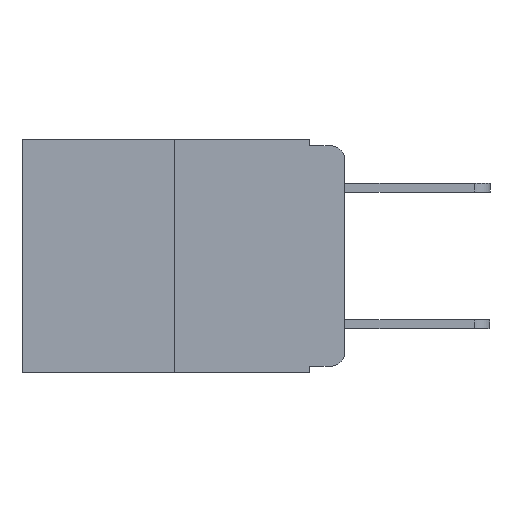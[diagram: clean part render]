
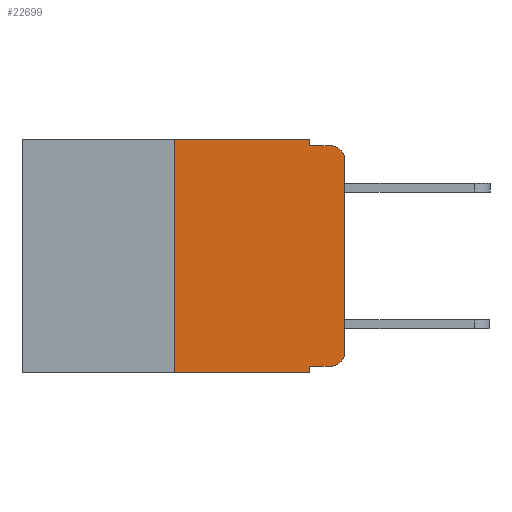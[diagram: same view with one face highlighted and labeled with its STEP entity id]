
A CAD part, left-side view. The second image highlights one B-rep face of the part: STEP entity #22699.
In plain terms, the highlighted planar face has unit normal (-1, 0, 0).
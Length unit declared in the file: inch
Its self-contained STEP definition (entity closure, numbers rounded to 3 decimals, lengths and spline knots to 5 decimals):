
#502 = DIRECTION ( 'NONE',  ( 0., -1., 0. ) ) ;
#968 = LINE ( 'NONE', #11239, #16253 ) ;
#1039 = CARTESIAN_POINT ( 'NONE',  ( 0., 0., -0.313 ) ) ;
#1352 = LINE ( 'NONE', #9816, #16007 ) ;
#1922 = LINE ( 'NONE', #12638, #11921 ) ;
#2007 = AXIS2_PLACEMENT_3D ( 'NONE', #10311, #23883, #12305 ) ;
#2706 = VECTOR ( 'NONE', #15380, 39.37008 ) ;
#2947 = ORIENTED_EDGE ( 'NONE', *, *, #20778, .T. ) ;
#3689 = VERTEX_POINT ( 'NONE', #8313 ) ;
#4048 = AXIS2_PLACEMENT_3D ( 'NONE', #19145, #7368, #21078 ) ;
#4637 = CARTESIAN_POINT ( 'NONE',  ( 0., 0.25, 0. ) ) ;
#5293 = LINE ( 'NONE', #9730, #15257 ) ;
#5774 = DIRECTION ( 'NONE',  ( 0., 0., -1. ) ) ;
#6338 = VERTEX_POINT ( 'NONE', #1039 ) ;
#7019 = ORIENTED_EDGE ( 'NONE', *, *, #24613, .T. ) ;
#7368 = DIRECTION ( 'NONE',  ( -1., 0., 0. ) ) ;
#7663 = EDGE_CURVE ( 'NONE', #12164, #6338, #9900, .T. ) ;
#8277 = EDGE_LOOP ( 'NONE', ( #7019, #2947, #14176, #24402, #10771, #17253, #13262, #8596, #19635, #24722 ) ) ;
#8313 = CARTESIAN_POINT ( 'NONE',  ( 0., 0.25, -0.343 ) ) ;
#8409 = VECTOR ( 'NONE', #10674, 39.37008 ) ;
#8506 = VERTEX_POINT ( 'NONE', #14765 ) ;
#8596 = ORIENTED_EDGE ( 'NONE', *, *, #14300, .F. ) ;
#8674 = VERTEX_POINT ( 'NONE', #11205 ) ;
#9271 = VECTOR ( 'NONE', #502, 39.37008 ) ;
#9400 = CARTESIAN_POINT ( 'NONE',  ( 0., 0., 0. ) ) ;
#9730 = CARTESIAN_POINT ( 'NONE',  ( 0., 0.473, 0. ) ) ;
#9816 = CARTESIAN_POINT ( 'NONE',  ( 0., 0.051, -0.333 ) ) ;
#9887 = LINE ( 'NONE', #12504, #9271 ) ;
#9900 = CIRCLE ( 'NONE', #2007, 0.02 ) ;
#10311 = CARTESIAN_POINT ( 'NONE',  ( 0., 0.02, -0.313 ) ) ;
#10498 = LINE ( 'NONE', #20859, #20245 ) ;
#10674 = DIRECTION ( 'NONE',  ( 0., 0., 1. ) ) ;
#10771 = ORIENTED_EDGE ( 'NONE', *, *, #15335, .F. ) ;
#11205 = CARTESIAN_POINT ( 'NONE',  ( 0., 0.051, -0.333 ) ) ;
#11239 = CARTESIAN_POINT ( 'NONE',  ( 0., 0.051, -0.01 ) ) ;
#11692 = CARTESIAN_POINT ( 'NONE',  ( 0., 0.473, 0. ) ) ;
#11721 = DIRECTION ( 'NONE',  ( 0., -1., 0. ) ) ;
#11921 = VECTOR ( 'NONE', #22449, 39.37008 ) ;
#12164 = VERTEX_POINT ( 'NONE', #17006 ) ;
#12305 = DIRECTION ( 'NONE',  ( 0., 0., -1. ) ) ;
#12504 = CARTESIAN_POINT ( 'NONE',  ( 0., 0.473, -0.343 ) ) ;
#12511 = CARTESIAN_POINT ( 'NONE',  ( 0., 0., -0.03 ) ) ;
#12638 = CARTESIAN_POINT ( 'NONE',  ( 0., 0.051, 0. ) ) ;
#12680 = VERTEX_POINT ( 'NONE', #12511 ) ;
#12684 = LINE ( 'NONE', #9400, #2706 ) ;
#12969 = EDGE_CURVE ( 'NONE', #8674, #12164, #1352, .T. ) ;
#13262 = ORIENTED_EDGE ( 'NONE', *, *, #24957, .T. ) ;
#13897 = VERTEX_POINT ( 'NONE', #17391 ) ;
#14028 = VERTEX_POINT ( 'NONE', #15843 ) ;
#14176 = ORIENTED_EDGE ( 'NONE', *, *, #19496, .F. ) ;
#14300 = EDGE_CURVE ( 'NONE', #8674, #8506, #1922, .T. ) ;
#14406 = VERTEX_POINT ( 'NONE', #22615 ) ;
#14765 = CARTESIAN_POINT ( 'NONE',  ( 0., 0.051, -0.343 ) ) ;
#15257 = VECTOR ( 'NONE', #11721, 39.37008 ) ;
#15335 = EDGE_CURVE ( 'NONE', #13897, #14406, #5293, .T. ) ;
#15380 = DIRECTION ( 'NONE',  ( 0., 0., 1. ) ) ;
#15629 = EDGE_CURVE ( 'NONE', #3689, #13897, #23933, .T. ) ;
#15679 = PLANE ( 'NONE',  #19598 ) ;
#15843 = CARTESIAN_POINT ( 'NONE',  ( 0., 0.051, -0.01 ) ) ;
#16007 = VECTOR ( 'NONE', #17735, 39.37008 ) ;
#16253 = VECTOR ( 'NONE', #22876, 39.37008 ) ;
#17006 = CARTESIAN_POINT ( 'NONE',  ( 0., 0.02, -0.333 ) ) ;
#17099 = FACE_OUTER_BOUND ( 'NONE', #8277, .T. ) ;
#17253 = ORIENTED_EDGE ( 'NONE', *, *, #15629, .F. ) ;
#17391 = CARTESIAN_POINT ( 'NONE',  ( 0., 0.25, 0. ) ) ;
#17631 = DIRECTION ( 'NONE',  ( 1., 0., 0. ) ) ;
#17735 = DIRECTION ( 'NONE',  ( 0., -1., 0. ) ) ;
#18222 = EDGE_CURVE ( 'NONE', #14406, #14028, #10498, .T. ) ;
#19145 = CARTESIAN_POINT ( 'NONE',  ( 0., 0.02, -0.03 ) ) ;
#19496 = EDGE_CURVE ( 'NONE', #14028, #23543, #968, .T. ) ;
#19598 = AXIS2_PLACEMENT_3D ( 'NONE', #11692, #17631, #5774 ) ;
#19635 = ORIENTED_EDGE ( 'NONE', *, *, #12969, .T. ) ;
#20169 = CARTESIAN_POINT ( 'NONE',  ( 0., 0.02, -0.01 ) ) ;
#20245 = VECTOR ( 'NONE', #22773, 39.37008 ) ;
#20778 = EDGE_CURVE ( 'NONE', #12680, #23543, #24265, .T. ) ;
#20859 = CARTESIAN_POINT ( 'NONE',  ( 0., 0.051, 0. ) ) ;
#21078 = DIRECTION ( 'NONE',  ( 0., 0., -1. ) ) ;
#22449 = DIRECTION ( 'NONE',  ( 0., 0., -1. ) ) ;
#22615 = CARTESIAN_POINT ( 'NONE',  ( 0., 0.051, 0. ) ) ;
#22699 = ADVANCED_FACE ( 'NONE', ( #17099 ), #15679, .F. ) ;
#22773 = DIRECTION ( 'NONE',  ( 0., 0., -1. ) ) ;
#22876 = DIRECTION ( 'NONE',  ( 0., -1., 0. ) ) ;
#23543 = VERTEX_POINT ( 'NONE', #20169 ) ;
#23883 = DIRECTION ( 'NONE',  ( -1., 0., 0. ) ) ;
#23933 = LINE ( 'NONE', #4637, #8409 ) ;
#24265 = CIRCLE ( 'NONE', #4048, 0.02 ) ;
#24402 = ORIENTED_EDGE ( 'NONE', *, *, #18222, .F. ) ;
#24613 = EDGE_CURVE ( 'NONE', #6338, #12680, #12684, .T. ) ;
#24722 = ORIENTED_EDGE ( 'NONE', *, *, #7663, .T. ) ;
#24957 = EDGE_CURVE ( 'NONE', #3689, #8506, #9887, .T. ) ;
